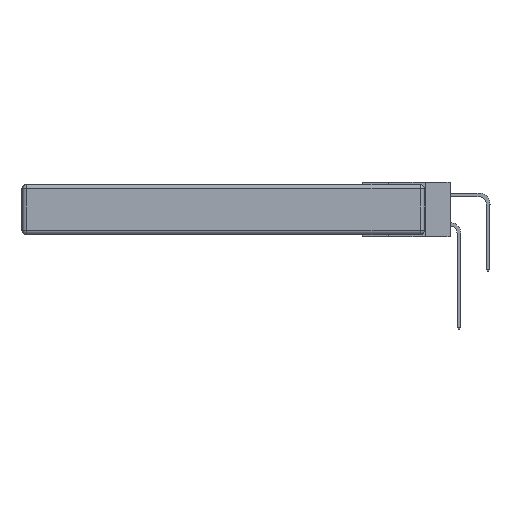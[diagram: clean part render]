
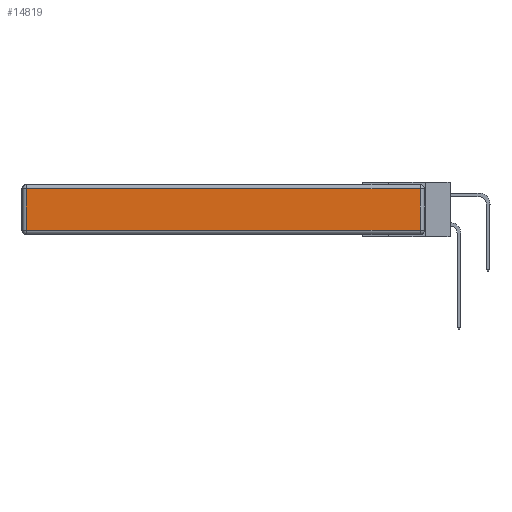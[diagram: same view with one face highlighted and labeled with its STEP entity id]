
A CAD part, left-side view. The second image highlights one B-rep face of the part: STEP entity #14819.
In plain terms, the highlighted planar face has unit normal (-1, 0, 0).
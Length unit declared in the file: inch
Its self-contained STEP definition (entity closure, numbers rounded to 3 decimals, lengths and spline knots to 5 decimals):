
#383 = PLANE ( 'NONE',  #35308 ) ;
#798 = ORIENTED_EDGE ( 'NONE', *, *, #26986, .T. ) ;
#1911 = CARTESIAN_POINT ( 'NONE',  ( 0., 0., -0.313 ) ) ;
#1938 = VERTEX_POINT ( 'NONE', #35563 ) ;
#5185 = LINE ( 'NONE', #19026, #25577 ) ;
#6781 = EDGE_LOOP ( 'NONE', ( #15664, #26846, #798, #26393 ) ) ;
#7680 = DIRECTION ( 'NONE',  ( 0., 1., 0. ) ) ;
#7971 = CARTESIAN_POINT ( 'NONE',  ( 0., 0.03, -0.343 ) ) ;
#8135 = CARTESIAN_POINT ( 'NONE',  ( 0., 2.72, -0.313 ) ) ;
#8262 = DIRECTION ( 'NONE',  ( 0., 0., -1. ) ) ;
#11793 = EDGE_CURVE ( 'NONE', #18085, #32498, #22271, .T. ) ;
#14683 = CARTESIAN_POINT ( 'NONE',  ( 0., 0.03, -0.313 ) ) ;
#14819 = ADVANCED_FACE ( 'NONE', ( #31618 ), #383, .T. ) ;
#15664 = ORIENTED_EDGE ( 'NONE', *, *, #11793, .T. ) ;
#16616 = VECTOR ( 'NONE', #21317, 39.37008 ) ;
#17102 = EDGE_CURVE ( 'NONE', #19894, #18085, #5185, .T. ) ;
#17110 = DIRECTION ( 'NONE',  ( 0., 0., 1. ) ) ;
#18085 = VERTEX_POINT ( 'NONE', #8135 ) ;
#18680 = CARTESIAN_POINT ( 'NONE',  ( 0., 2.75, -0.03 ) ) ;
#19026 = CARTESIAN_POINT ( 'NONE',  ( 0., 2.72, -0.343 ) ) ;
#19466 = DIRECTION ( 'NONE',  ( 0., 0., 1. ) ) ;
#19785 = DIRECTION ( 'NONE',  ( -1., 0., 0. ) ) ;
#19894 = VERTEX_POINT ( 'NONE', #34884 ) ;
#21317 = DIRECTION ( 'NONE',  ( 0., -1., 0. ) ) ;
#22271 = LINE ( 'NONE', #1911, #16616 ) ;
#25577 = VECTOR ( 'NONE', #8262, 39.37008 ) ;
#26048 = LINE ( 'NONE', #7971, #29538 ) ;
#26164 = VECTOR ( 'NONE', #7680, 39.37008 ) ;
#26393 = ORIENTED_EDGE ( 'NONE', *, *, #17102, .T. ) ;
#26622 = LINE ( 'NONE', #18680, #26164 ) ;
#26846 = ORIENTED_EDGE ( 'NONE', *, *, #31652, .T. ) ;
#26986 = EDGE_CURVE ( 'NONE', #1938, #19894, #26622, .T. ) ;
#28185 = CARTESIAN_POINT ( 'NONE',  ( 0., 0., -0.343 ) ) ;
#29538 = VECTOR ( 'NONE', #19466, 39.37008 ) ;
#31618 = FACE_OUTER_BOUND ( 'NONE', #6781, .T. ) ;
#31652 = EDGE_CURVE ( 'NONE', #32498, #1938, #26048, .T. ) ;
#32498 = VERTEX_POINT ( 'NONE', #14683 ) ;
#34884 = CARTESIAN_POINT ( 'NONE',  ( 0., 2.72, -0.03 ) ) ;
#35308 = AXIS2_PLACEMENT_3D ( 'NONE', #28185, #19785, #17110 ) ;
#35563 = CARTESIAN_POINT ( 'NONE',  ( 0., 0.03, -0.03 ) ) ;
